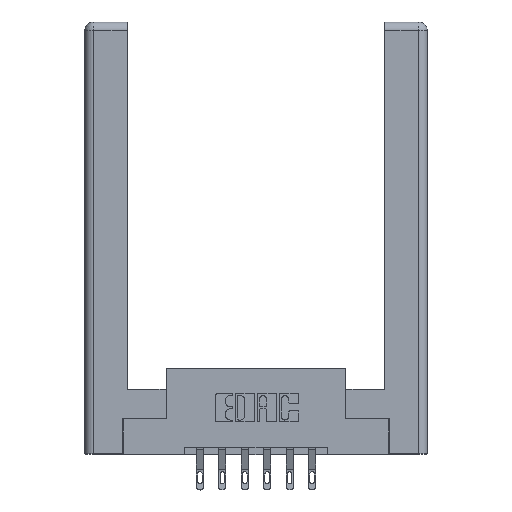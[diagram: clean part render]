
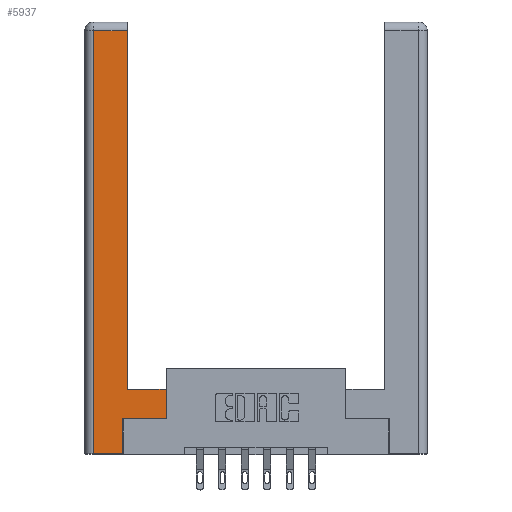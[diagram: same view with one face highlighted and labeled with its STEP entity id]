
A CAD part, top view. The second image highlights one B-rep face of the part: STEP entity #5937.
In plain terms, the highlighted planar face has unit normal (0, 0, 1).
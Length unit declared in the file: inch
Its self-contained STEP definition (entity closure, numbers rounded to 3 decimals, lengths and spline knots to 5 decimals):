
#14 = EDGE_CURVE ( 'NONE', #8255, #3394, #2148, .T. ) ;
#84 = DIRECTION ( 'NONE',  ( -1., 0., 0. ) ) ;
#186 = LINE ( 'NONE', #9801, #5797 ) ;
#264 = LINE ( 'NONE', #10943, #5405 ) ;
#620 = CARTESIAN_POINT ( 'NONE',  ( 0., 0., 0. ) ) ;
#769 = EDGE_CURVE ( 'NONE', #3619, #2596, #9250, .T. ) ;
#970 = CARTESIAN_POINT ( 'NONE',  ( 0.265, 0., 0. ) ) ;
#1237 = CARTESIAN_POINT ( 'NONE',  ( 0.295, 0.45, 0. ) ) ;
#1421 = CARTESIAN_POINT ( 'NONE',  ( 0.295, 2.94, 0. ) ) ;
#1510 = DIRECTION ( 'NONE',  ( 0., 0., -1. ) ) ;
#1550 = PLANE ( 'NONE',  #1752 ) ;
#1752 = AXIS2_PLACEMENT_3D ( 'NONE', #620, #1510, #7191 ) ;
#1941 = VECTOR ( 'NONE', #4518, 39.37008 ) ;
#2007 = EDGE_CURVE ( 'NONE', #5859, #4656, #8348, .T. ) ;
#2101 = CARTESIAN_POINT ( 'NONE',  ( 0.0615, 2.94, 0. ) ) ;
#2148 = LINE ( 'NONE', #4222, #3922 ) ;
#2268 = CARTESIAN_POINT ( 'NONE',  ( 0.0615, 2.94, 0. ) ) ;
#2465 = EDGE_CURVE ( 'NONE', #2596, #5859, #12178, .T. ) ;
#2596 = VERTEX_POINT ( 'NONE', #1421 ) ;
#2616 = CARTESIAN_POINT ( 'NONE',  ( 0.295, 3., 0. ) ) ;
#3293 = DIRECTION ( 'NONE',  ( 0., 1., 0. ) ) ;
#3394 = VERTEX_POINT ( 'NONE', #5014 ) ;
#3487 = LINE ( 'NONE', #12254, #4523 ) ;
#3555 = DIRECTION ( 'NONE',  ( 0., 1., 0. ) ) ;
#3619 = VERTEX_POINT ( 'NONE', #9317 ) ;
#3650 = VERTEX_POINT ( 'NONE', #970 ) ;
#3922 = VECTOR ( 'NONE', #3293, 39.37008 ) ;
#3973 = DIRECTION ( 'NONE',  ( 1., 0., 0. ) ) ;
#4138 = EDGE_CURVE ( 'NONE', #3650, #9357, #186, .T. ) ;
#4170 = LINE ( 'NONE', #1237, #8206 ) ;
#4222 = CARTESIAN_POINT ( 'NONE',  ( 0.565, 0.45, 0. ) ) ;
#4518 = DIRECTION ( 'NONE',  ( 0., -1., 0. ) ) ;
#4523 = VECTOR ( 'NONE', #3973, 39.37008 ) ;
#4656 = VERTEX_POINT ( 'NONE', #7365 ) ;
#5014 = CARTESIAN_POINT ( 'NONE',  ( 0.565, 0.45, 0. ) ) ;
#5061 = VECTOR ( 'NONE', #3555, 39.37008 ) ;
#5190 = DIRECTION ( 'NONE',  ( -1., 0., 0. ) ) ;
#5405 = VECTOR ( 'NONE', #12138, 39.37008 ) ;
#5430 = ORIENTED_EDGE ( 'NONE', *, *, #14, .T. ) ;
#5797 = VECTOR ( 'NONE', #11911, 39.37008 ) ;
#5859 = VERTEX_POINT ( 'NONE', #2268 ) ;
#5867 = ORIENTED_EDGE ( 'NONE', *, *, #7833, .T. ) ;
#5937 = ADVANCED_FACE ( 'NONE', ( #6412 ), #1550, .F. ) ;
#6030 = ORIENTED_EDGE ( 'NONE', *, *, #4138, .T. ) ;
#6412 = FACE_OUTER_BOUND ( 'NONE', #9903, .T. ) ;
#6445 = EDGE_CURVE ( 'NONE', #3394, #3619, #4170, .T. ) ;
#6592 = ORIENTED_EDGE ( 'NONE', *, *, #6445, .T. ) ;
#7149 = EDGE_CURVE ( 'NONE', #9357, #8255, #3487, .T. ) ;
#7191 = DIRECTION ( 'NONE',  ( -1., 0., 0. ) ) ;
#7365 = CARTESIAN_POINT ( 'NONE',  ( 0.0615, 0., 0. ) ) ;
#7437 = VECTOR ( 'NONE', #84, 39.37008 ) ;
#7547 = CARTESIAN_POINT ( 'NONE',  ( 0.565, 0.245, 0. ) ) ;
#7833 = EDGE_CURVE ( 'NONE', #4656, #3650, #264, .T. ) ;
#8206 = VECTOR ( 'NONE', #5190, 39.37008 ) ;
#8255 = VERTEX_POINT ( 'NONE', #7547 ) ;
#8348 = LINE ( 'NONE', #12219, #1941 ) ;
#8898 = ORIENTED_EDGE ( 'NONE', *, *, #2465, .T. ) ;
#9250 = LINE ( 'NONE', #2616, #5061 ) ;
#9268 = ORIENTED_EDGE ( 'NONE', *, *, #769, .T. ) ;
#9317 = CARTESIAN_POINT ( 'NONE',  ( 0.295, 0.45, 0. ) ) ;
#9357 = VERTEX_POINT ( 'NONE', #9791 ) ;
#9791 = CARTESIAN_POINT ( 'NONE',  ( 0.265, 0.245, 0. ) ) ;
#9801 = CARTESIAN_POINT ( 'NONE',  ( 0.265, 0.245, 0. ) ) ;
#9825 = ORIENTED_EDGE ( 'NONE', *, *, #7149, .T. ) ;
#9903 = EDGE_LOOP ( 'NONE', ( #9268, #8898, #12121, #5867, #6030, #9825, #5430, #6592 ) ) ;
#10943 = CARTESIAN_POINT ( 'NONE',  ( 0.265, 0., 0. ) ) ;
#11911 = DIRECTION ( 'NONE',  ( 0., 1., 0. ) ) ;
#12121 = ORIENTED_EDGE ( 'NONE', *, *, #2007, .T. ) ;
#12138 = DIRECTION ( 'NONE',  ( 1., 0., 0. ) ) ;
#12178 = LINE ( 'NONE', #2101, #7437 ) ;
#12219 = CARTESIAN_POINT ( 'NONE',  ( 0.0615, 0., 0. ) ) ;
#12254 = CARTESIAN_POINT ( 'NONE',  ( 0.565, 0.245, 0. ) ) ;
